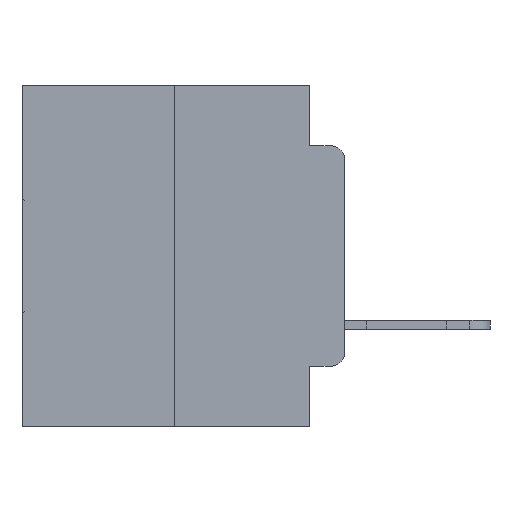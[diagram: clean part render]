
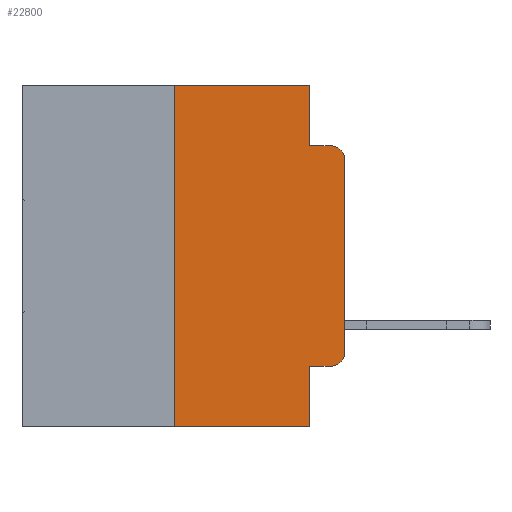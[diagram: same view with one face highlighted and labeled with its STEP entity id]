
A CAD part, left-side view. The second image highlights one B-rep face of the part: STEP entity #22800.
In plain terms, the highlighted planar face has unit normal (-1, 0, 0).
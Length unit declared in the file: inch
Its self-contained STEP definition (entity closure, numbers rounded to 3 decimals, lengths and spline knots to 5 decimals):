
#263 = LINE ( 'NONE', #27268, #6565 ) ;
#1780 = AXIS2_PLACEMENT_3D ( 'NONE', #27559, #25339, #11320 ) ;
#2347 = ORIENTED_EDGE ( 'NONE', *, *, #7211, .F. ) ;
#2383 = VECTOR ( 'NONE', #22770, 39.37008 ) ;
#2779 = LINE ( 'NONE', #13215, #29198 ) ;
#3250 = LINE ( 'NONE', #23265, #2383 ) ;
#4378 = VECTOR ( 'NONE', #21569, 39.37008 ) ;
#5326 = VERTEX_POINT ( 'NONE', #17364 ) ;
#5366 = CARTESIAN_POINT ( 'NONE',  ( 0., 0.02, -0.4115 ) ) ;
#6527 = LINE ( 'NONE', #10841, #30786 ) ;
#6565 = VECTOR ( 'NONE', #27054, 39.37008 ) ;
#6574 = ORIENTED_EDGE ( 'NONE', *, *, #22328, .T. ) ;
#6931 = DIRECTION ( 'NONE',  ( -1., 0., 0. ) ) ;
#7060 = CARTESIAN_POINT ( 'NONE',  ( 0., 0.02, -0.1085 ) ) ;
#7160 = CARTESIAN_POINT ( 'NONE',  ( 0., 0.051, -0.4115 ) ) ;
#7211 = EDGE_CURVE ( 'NONE', #13499, #5326, #2779, .T. ) ;
#7314 = VERTEX_POINT ( 'NONE', #12147 ) ;
#8034 = CARTESIAN_POINT ( 'NONE',  ( 0., 0.051, -0.0885 ) ) ;
#8725 = PLANE ( 'NONE',  #1780 ) ;
#9106 = AXIS2_PLACEMENT_3D ( 'NONE', #7060, #23874, #9685 ) ;
#9406 = ORIENTED_EDGE ( 'NONE', *, *, #13177, .T. ) ;
#9592 = VECTOR ( 'NONE', #11701, 39.37008 ) ;
#9685 = DIRECTION ( 'NONE',  ( 0., 0., -1. ) ) ;
#10173 = VERTEX_POINT ( 'NONE', #29070 ) ;
#10756 = VECTOR ( 'NONE', #15154, 39.37008 ) ;
#10841 = CARTESIAN_POINT ( 'NONE',  ( 0., 0., 0. ) ) ;
#11022 = ORIENTED_EDGE ( 'NONE', *, *, #26977, .F. ) ;
#11110 = VERTEX_POINT ( 'NONE', #30688 ) ;
#11320 = DIRECTION ( 'NONE',  ( 0., 0., -1. ) ) ;
#11490 = VERTEX_POINT ( 'NONE', #8034 ) ;
#11701 = DIRECTION ( 'NONE',  ( 0., 0., -1. ) ) ;
#11859 = AXIS2_PLACEMENT_3D ( 'NONE', #21378, #6931, #23742 ) ;
#12147 = CARTESIAN_POINT ( 'NONE',  ( 0., 0.051, -0.5 ) ) ;
#12170 = CARTESIAN_POINT ( 'NONE',  ( 0., 0.051, 0. ) ) ;
#13173 = DIRECTION ( 'NONE',  ( 0., 0., 1. ) ) ;
#13177 = EDGE_CURVE ( 'NONE', #13499, #7314, #263, .T. ) ;
#13215 = CARTESIAN_POINT ( 'NONE',  ( 0., 0.25, 0. ) ) ;
#13302 = VERTEX_POINT ( 'NONE', #21753 ) ;
#13499 = VERTEX_POINT ( 'NONE', #15190 ) ;
#13739 = CIRCLE ( 'NONE', #11859, 0.02 ) ;
#13965 = EDGE_CURVE ( 'NONE', #14142, #11490, #26522, .T. ) ;
#14142 = VERTEX_POINT ( 'NONE', #12170 ) ;
#15154 = DIRECTION ( 'NONE',  ( 0., -1., 0. ) ) ;
#15190 = CARTESIAN_POINT ( 'NONE',  ( 0., 0.25, -0.5 ) ) ;
#15475 = EDGE_CURVE ( 'NONE', #11490, #13302, #3250, .T. ) ;
#17364 = CARTESIAN_POINT ( 'NONE',  ( 0., 0.25, 0. ) ) ;
#17402 = EDGE_LOOP ( 'NONE', ( #23122, #17654, #29846, #25321, #31142, #2347, #9406, #11022, #24973, #6574 ) ) ;
#17572 = LINE ( 'NONE', #7160, #4378 ) ;
#17654 = ORIENTED_EDGE ( 'NONE', *, *, #18653, .T. ) ;
#18653 = EDGE_CURVE ( 'NONE', #10173, #13302, #27327, .T. ) ;
#19638 = VECTOR ( 'NONE', #28190, 39.37008 ) ;
#19789 = CARTESIAN_POINT ( 'NONE',  ( 0., 0.473, 0. ) ) ;
#20590 = EDGE_CURVE ( 'NONE', #5326, #14142, #24020, .T. ) ;
#20856 = CARTESIAN_POINT ( 'NONE',  ( 0., 0., -0.3915 ) ) ;
#21378 = CARTESIAN_POINT ( 'NONE',  ( 0., 0.02, -0.3915 ) ) ;
#21467 = LINE ( 'NONE', #28023, #9592 ) ;
#21569 = DIRECTION ( 'NONE',  ( 0., -1., 0. ) ) ;
#21753 = CARTESIAN_POINT ( 'NONE',  ( 0., 0.02, -0.0885 ) ) ;
#21974 = VERTEX_POINT ( 'NONE', #5366 ) ;
#22328 = EDGE_CURVE ( 'NONE', #21974, #28926, #13739, .T. ) ;
#22770 = DIRECTION ( 'NONE',  ( 0., -1., 0. ) ) ;
#22800 = ADVANCED_FACE ( 'NONE', ( #28496 ), #8725, .F. ) ;
#23122 = ORIENTED_EDGE ( 'NONE', *, *, #23305, .T. ) ;
#23265 = CARTESIAN_POINT ( 'NONE',  ( 0., 0.051, -0.0885 ) ) ;
#23305 = EDGE_CURVE ( 'NONE', #28926, #10173, #6527, .T. ) ;
#23742 = DIRECTION ( 'NONE',  ( 0., 0., -1. ) ) ;
#23874 = DIRECTION ( 'NONE',  ( -1., 0., 0. ) ) ;
#23904 = EDGE_CURVE ( 'NONE', #11110, #21974, #17572, .T. ) ;
#24020 = LINE ( 'NONE', #19789, #10756 ) ;
#24973 = ORIENTED_EDGE ( 'NONE', *, *, #23904, .T. ) ;
#25321 = ORIENTED_EDGE ( 'NONE', *, *, #13965, .F. ) ;
#25339 = DIRECTION ( 'NONE',  ( 1., 0., 0. ) ) ;
#26522 = LINE ( 'NONE', #27576, #19638 ) ;
#26977 = EDGE_CURVE ( 'NONE', #11110, #7314, #21467, .T. ) ;
#27054 = DIRECTION ( 'NONE',  ( 0., -1., 0. ) ) ;
#27213 = DIRECTION ( 'NONE',  ( 0., 0., 1. ) ) ;
#27268 = CARTESIAN_POINT ( 'NONE',  ( 0., 0.473, -0.5 ) ) ;
#27327 = CIRCLE ( 'NONE', #9106, 0.02 ) ;
#27559 = CARTESIAN_POINT ( 'NONE',  ( 0., 0.473, 0. ) ) ;
#27576 = CARTESIAN_POINT ( 'NONE',  ( 0., 0.051, 0. ) ) ;
#28023 = CARTESIAN_POINT ( 'NONE',  ( 0., 0.051, 0. ) ) ;
#28190 = DIRECTION ( 'NONE',  ( 0., 0., -1. ) ) ;
#28496 = FACE_OUTER_BOUND ( 'NONE', #17402, .T. ) ;
#28926 = VERTEX_POINT ( 'NONE', #20856 ) ;
#29070 = CARTESIAN_POINT ( 'NONE',  ( 0., 0., -0.1085 ) ) ;
#29198 = VECTOR ( 'NONE', #13173, 39.37008 ) ;
#29846 = ORIENTED_EDGE ( 'NONE', *, *, #15475, .F. ) ;
#30688 = CARTESIAN_POINT ( 'NONE',  ( 0., 0.051, -0.4115 ) ) ;
#30786 = VECTOR ( 'NONE', #27213, 39.37008 ) ;
#31142 = ORIENTED_EDGE ( 'NONE', *, *, #20590, .F. ) ;
